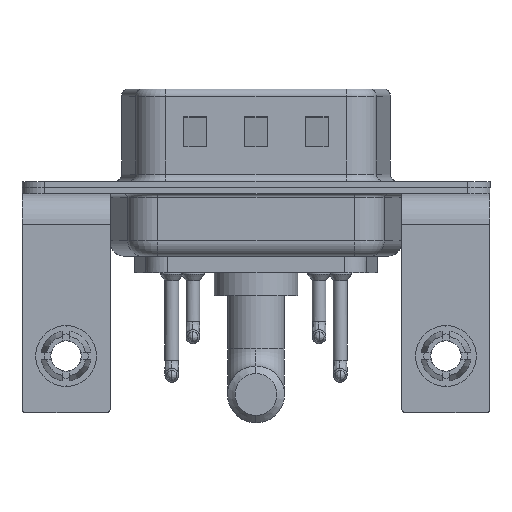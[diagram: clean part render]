
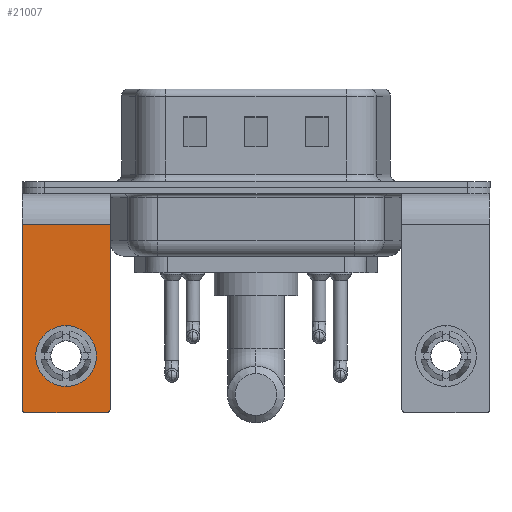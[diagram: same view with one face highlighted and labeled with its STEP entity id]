
A CAD part, front view. The second image highlights one B-rep face of the part: STEP entity #21007.
In plain terms, the highlighted planar face has unit normal (0, -1, 0).
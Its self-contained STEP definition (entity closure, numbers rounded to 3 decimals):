
#32 = AXIS2_PLACEMENT_3D ( 'NONE', #19515, #2763, #16202 ) ;
#151 = VECTOR ( 'NONE', #16326, 1000. ) ;
#202 = CARTESIAN_POINT ( 'NONE',  ( -2.9, -6.25, -14.55 ) ) ;
#310 = LINE ( 'NONE', #3503, #9824 ) ;
#477 = ORIENTED_EDGE ( 'NONE', *, *, #10059, .T. ) ;
#803 = AXIS2_PLACEMENT_3D ( 'NONE', #15444, #16901, #13460 ) ;
#932 = AXIS2_PLACEMENT_3D ( 'NONE', #14215, #17646, #21076 ) ;
#1299 = VECTOR ( 'NONE', #18534, 1000. ) ;
#1577 = EDGE_CURVE ( 'NONE', #8963, #13987, #2457, .T. ) ;
#1770 = EDGE_CURVE ( 'NONE', #19063, #13987, #10753, .T. ) ;
#1772 = LINE ( 'NONE', #20181, #1299 ) ;
#1901 = FACE_BOUND ( 'NONE', #21230, .T. ) ;
#2457 = LINE ( 'NONE', #4125, #151 ) ;
#2709 = AXIS2_PLACEMENT_3D ( 'NONE', #15509, #12292, #3526 ) ;
#2763 = DIRECTION ( 'NONE',  ( 0., 1., 0. ) ) ;
#2893 = DIRECTION ( 'NONE',  ( 0., -1., 0. ) ) ;
#3503 = CARTESIAN_POINT ( 'NONE',  ( 2.9, -6.25, -2.4 ) ) ;
#3526 = DIRECTION ( 'NONE',  ( 0., 0., 1. ) ) ;
#3788 = CARTESIAN_POINT ( 'NONE',  ( 0., -6.25, -13.07 ) ) ;
#4125 = CARTESIAN_POINT ( 'NONE',  ( 2.9, -6.25, -14.8 ) ) ;
#4407 = ORIENTED_EDGE ( 'NONE', *, *, #19667, .T. ) ;
#4478 = VERTEX_POINT ( 'NONE', #3788 ) ;
#4558 = CARTESIAN_POINT ( 'NONE',  ( -2.65, -6.25, -14.55 ) ) ;
#6550 = DIRECTION ( 'NONE',  ( 0., 0., 1. ) ) ;
#6686 = FACE_OUTER_BOUND ( 'NONE', #21616, .T. ) ;
#8583 = CARTESIAN_POINT ( 'NONE',  ( 0., -6.25, -9.07 ) ) ;
#8963 = VERTEX_POINT ( 'NONE', #21270 ) ;
#9440 = CIRCLE ( 'NONE', #2709, 2. ) ;
#9824 = VECTOR ( 'NONE', #13822, 1000. ) ;
#10059 = EDGE_CURVE ( 'NONE', #17166, #19063, #15921, .T. ) ;
#10211 = EDGE_CURVE ( 'NONE', #18417, #12773, #1772, .T. ) ;
#10753 = CIRCLE ( 'NONE', #12184, 0.25 ) ;
#11545 = CIRCLE ( 'NONE', #932, 0.25 ) ;
#11971 = ORIENTED_EDGE ( 'NONE', *, *, #12825, .T. ) ;
#12184 = AXIS2_PLACEMENT_3D ( 'NONE', #4558, #2893, #6550 ) ;
#12292 = DIRECTION ( 'NONE',  ( 0., 1., 0. ) ) ;
#12773 = VERTEX_POINT ( 'NONE', #17002 ) ;
#12825 = EDGE_CURVE ( 'NONE', #8963, #12773, #11545, .T. ) ;
#12895 = CARTESIAN_POINT ( 'NONE',  ( 2.9, -6.25, -2.4 ) ) ;
#13326 = ORIENTED_EDGE ( 'NONE', *, *, #1770, .T. ) ;
#13460 = DIRECTION ( 'NONE',  ( 0., 0., 1. ) ) ;
#13721 = EDGE_CURVE ( 'NONE', #14670, #4478, #9440, .T. ) ;
#13822 = DIRECTION ( 'NONE',  ( -1., 0., 0. ) ) ;
#13987 = VERTEX_POINT ( 'NONE', #14712 ) ;
#14157 = EDGE_CURVE ( 'NONE', #18417, #17166, #310, .T. ) ;
#14215 = CARTESIAN_POINT ( 'NONE',  ( 2.65, -6.25, -14.55 ) ) ;
#14670 = VERTEX_POINT ( 'NONE', #8583 ) ;
#14712 = CARTESIAN_POINT ( 'NONE',  ( -2.65, -6.25, -14.8 ) ) ;
#15444 = CARTESIAN_POINT ( 'NONE',  ( 2.9, -6.25, -2.4 ) ) ;
#15509 = CARTESIAN_POINT ( 'NONE',  ( 0., -6.25, -11.07 ) ) ;
#15921 = LINE ( 'NONE', #17801, #16874 ) ;
#16202 = DIRECTION ( 'NONE',  ( 0., 0., 1. ) ) ;
#16326 = DIRECTION ( 'NONE',  ( -1., 0., 0. ) ) ;
#16874 = VECTOR ( 'NONE', #19128, 1000. ) ;
#16901 = DIRECTION ( 'NONE',  ( 0., 1., 0. ) ) ;
#17002 = CARTESIAN_POINT ( 'NONE',  ( 2.9, -6.25, -14.55 ) ) ;
#17166 = VERTEX_POINT ( 'NONE', #18036 ) ;
#17362 = CIRCLE ( 'NONE', #32, 2. ) ;
#17555 = ORIENTED_EDGE ( 'NONE', *, *, #10211, .F. ) ;
#17646 = DIRECTION ( 'NONE',  ( 0., -1., 0. ) ) ;
#17801 = CARTESIAN_POINT ( 'NONE',  ( -2.9, -6.25, -2.4 ) ) ;
#18036 = CARTESIAN_POINT ( 'NONE',  ( -2.9, -6.25, -2.4 ) ) ;
#18417 = VERTEX_POINT ( 'NONE', #12895 ) ;
#18534 = DIRECTION ( 'NONE',  ( 0., 0., -1. ) ) ;
#19034 = ORIENTED_EDGE ( 'NONE', *, *, #13721, .T. ) ;
#19063 = VERTEX_POINT ( 'NONE', #202 ) ;
#19128 = DIRECTION ( 'NONE',  ( 0., 0., -1. ) ) ;
#19515 = CARTESIAN_POINT ( 'NONE',  ( 0., -6.25, -11.07 ) ) ;
#19667 = EDGE_CURVE ( 'NONE', #4478, #14670, #17362, .T. ) ;
#20111 = PLANE ( 'NONE',  #803 ) ;
#20181 = CARTESIAN_POINT ( 'NONE',  ( 2.9, -6.25, -2.4 ) ) ;
#20280 = ORIENTED_EDGE ( 'NONE', *, *, #14157, .T. ) ;
#21007 = ADVANCED_FACE ( 'NONE', ( #1901, #6686 ), #20111, .F. ) ;
#21076 = DIRECTION ( 'NONE',  ( 0., 0., 1. ) ) ;
#21230 = EDGE_LOOP ( 'NONE', ( #4407, #19034 ) ) ;
#21270 = CARTESIAN_POINT ( 'NONE',  ( 2.65, -6.25, -14.8 ) ) ;
#21616 = EDGE_LOOP ( 'NONE', ( #477, #13326, #21753, #11971, #17555, #20280 ) ) ;
#21753 = ORIENTED_EDGE ( 'NONE', *, *, #1577, .F. ) ;
